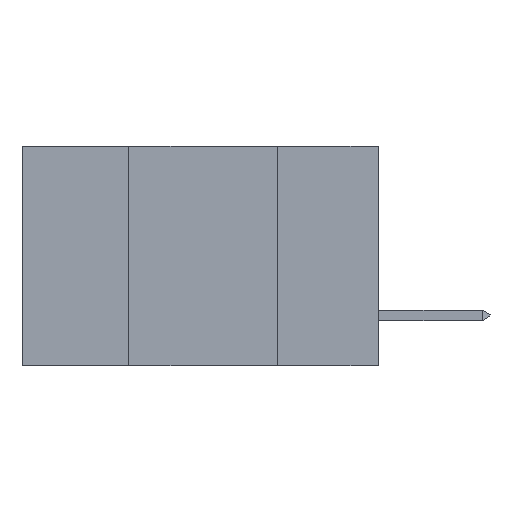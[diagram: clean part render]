
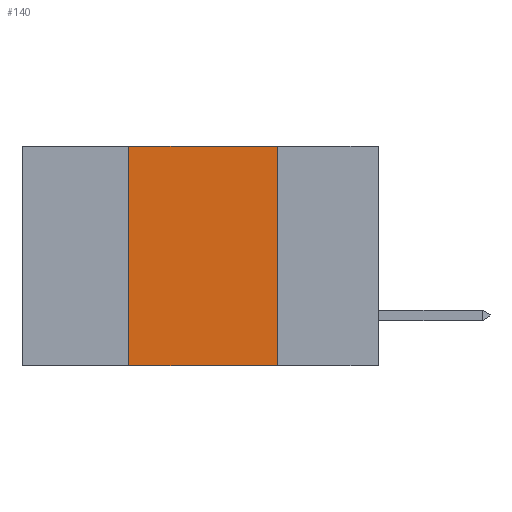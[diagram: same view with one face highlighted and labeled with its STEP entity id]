
A CAD part, left-side view. The second image highlights one B-rep face of the part: STEP entity #140.
In plain terms, the highlighted planar face has unit normal (-1, 0, 0).
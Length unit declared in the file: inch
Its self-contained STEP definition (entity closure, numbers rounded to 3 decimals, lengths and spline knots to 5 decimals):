
#78 = DIRECTION ( 'NONE',  ( 0., -1., 0. ) ) ;
#140 = ADVANCED_FACE ( 'NONE', ( #10031 ), #3304, .F. ) ;
#324 = EDGE_CURVE ( 'NONE', #679, #5605, #12380, .T. ) ;
#642 = AXIS2_PLACEMENT_3D ( 'NONE', #7173, #6290, #2248 ) ;
#679 = VERTEX_POINT ( 'NONE', #8080 ) ;
#785 = LINE ( 'NONE', #3104, #5710 ) ;
#1113 = CARTESIAN_POINT ( 'NONE',  ( 0., 0.6, 0. ) ) ;
#1346 = DIRECTION ( 'NONE',  ( 0., 0., -1. ) ) ;
#1428 = VERTEX_POINT ( 'NONE', #10784 ) ;
#2248 = DIRECTION ( 'NONE',  ( 0., 0., -1. ) ) ;
#2879 = ORIENTED_EDGE ( 'NONE', *, *, #7115, .F. ) ;
#3104 = CARTESIAN_POINT ( 'NONE',  ( 0., 0.6, -0.37 ) ) ;
#3304 = PLANE ( 'NONE',  #642 ) ;
#3370 = VECTOR ( 'NONE', #10470, 39.37008 ) ;
#3797 = EDGE_CURVE ( 'NONE', #1428, #7937, #9278, .T. ) ;
#3872 = ORIENTED_EDGE ( 'NONE', *, *, #9853, .T. ) ;
#4876 = LINE ( 'NONE', #1113, #11919 ) ;
#5605 = VERTEX_POINT ( 'NONE', #7291 ) ;
#5710 = VECTOR ( 'NONE', #8772, 39.37008 ) ;
#6290 = DIRECTION ( 'NONE',  ( 1., 0., 0. ) ) ;
#7115 = EDGE_CURVE ( 'NONE', #5605, #1428, #4876, .T. ) ;
#7173 = CARTESIAN_POINT ( 'NONE',  ( 0., 0.6, 0. ) ) ;
#7291 = CARTESIAN_POINT ( 'NONE',  ( 0., 0.42, 0. ) ) ;
#7937 = VERTEX_POINT ( 'NONE', #9979 ) ;
#8080 = CARTESIAN_POINT ( 'NONE',  ( 0., 0.42, -0.37 ) ) ;
#8418 = VECTOR ( 'NONE', #1346, 39.37008 ) ;
#8772 = DIRECTION ( 'NONE',  ( 0., -1., 0. ) ) ;
#8905 = EDGE_LOOP ( 'NONE', ( #10543, #2879, #12874, #3872 ) ) ;
#9278 = LINE ( 'NONE', #10192, #8418 ) ;
#9853 = EDGE_CURVE ( 'NONE', #679, #7937, #785, .T. ) ;
#9979 = CARTESIAN_POINT ( 'NONE',  ( 0., 0.17, -0.37 ) ) ;
#10031 = FACE_OUTER_BOUND ( 'NONE', #8905, .T. ) ;
#10192 = CARTESIAN_POINT ( 'NONE',  ( 0., 0.17, -0.37 ) ) ;
#10470 = DIRECTION ( 'NONE',  ( 0., 0., 1. ) ) ;
#10541 = CARTESIAN_POINT ( 'NONE',  ( 0., 0.42, -0.37 ) ) ;
#10543 = ORIENTED_EDGE ( 'NONE', *, *, #3797, .F. ) ;
#10784 = CARTESIAN_POINT ( 'NONE',  ( 0., 0.17, 0. ) ) ;
#11919 = VECTOR ( 'NONE', #78, 39.37008 ) ;
#12380 = LINE ( 'NONE', #10541, #3370 ) ;
#12874 = ORIENTED_EDGE ( 'NONE', *, *, #324, .F. ) ;
